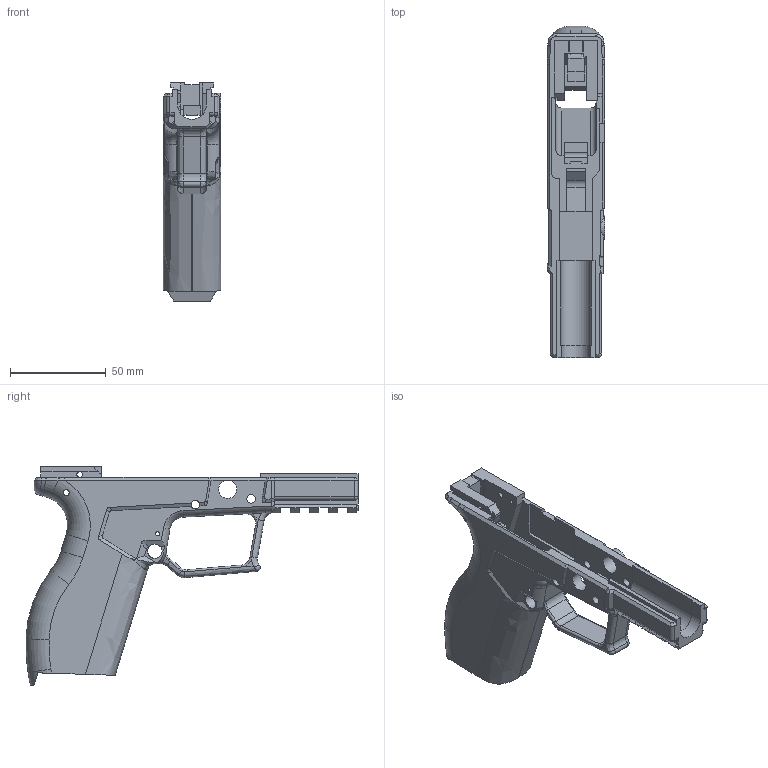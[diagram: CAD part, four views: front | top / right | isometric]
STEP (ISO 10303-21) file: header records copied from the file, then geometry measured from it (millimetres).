
FILE_DESCRIPTION(/* description */ (''),/* implementation_level */ '2;1');
FILE_NAME(/* name */ 'XD_ServiceSize_RC031322.step',/* time_stamp */ '2022-03-13T19:20:34-04:00',/* author */ (''),/* organization */ (''),/* preprocessor_version */ 'ST-DEVELOPER v18.1',/* originating_system */ 'Autodesk Translation Framework v10.13.0.1454',/* authorisation */ '');
FILE_SCHEMA (('AUTOMOTIVE_DESIGN { 1 0 10303 214 3 1 1 }'));
Length unit declared in the file: millimetre
Products named in the file (1): XD_ServiceSize
Bounding box: 30.25 x 173.2 x 113.92 mm (x, y, z)
Volume: 99386.8 mm3; surface area: 47064 mm2
Topology: 1 solids, 1 shells, 382 faces, 1100 edges, 699 vertices
Faces by surface type: plane 227, cylinder 76, bspline 50, torus 22, cone 5, sphere 2
Full cylindrical faces by diameter (mm): 2 x1, 2.15 x2, 3 x2, 3.15 x2, 4.5 x4, 7.5 x1, 9.5 x2
Entity records: 15212 total; most frequent: CARTESIAN_POINT 5355, ORIENTED_EDGE 2196, DIRECTION 1868, EDGE_CURVE 1098, LINE 726, VECTOR 726, VERTEX_POINT 699, AXIS2_PLACEMENT_3D 571
